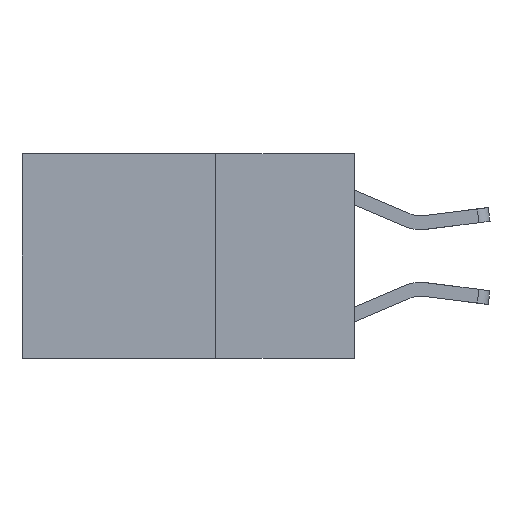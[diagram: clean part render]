
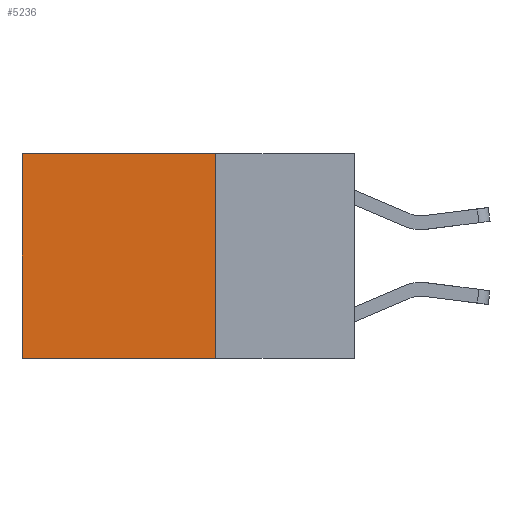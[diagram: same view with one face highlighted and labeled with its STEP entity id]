
A CAD part, left-side view. The second image highlights one B-rep face of the part: STEP entity #5236.
In plain terms, the highlighted planar face has unit normal (-1, 0, 0).
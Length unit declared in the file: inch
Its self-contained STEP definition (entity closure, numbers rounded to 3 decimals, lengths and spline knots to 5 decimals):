
#697 = DIRECTION ( 'NONE',  ( 0., 0., -1. ) ) ;
#700 = CARTESIAN_POINT ( 'NONE',  ( 0.2625, 0.25, 0. ) ) ;
#1028 = CARTESIAN_POINT ( 'NONE',  ( 0.2625, 0.25, 0. ) ) ;
#1201 = ORIENTED_EDGE ( 'NONE', *, *, #4564, .T. ) ;
#1416 = VERTEX_POINT ( 'NONE', #5200 ) ;
#1940 = ORIENTED_EDGE ( 'NONE', *, *, #8384, .F. ) ;
#2010 = VECTOR ( 'NONE', #697, 39.37008 ) ;
#2042 = AXIS2_PLACEMENT_3D ( 'NONE', #700, #9902, #4438 ) ;
#3143 = VECTOR ( 'NONE', #3541, 39.37008 ) ;
#3192 = LINE ( 'NONE', #9416, #2010 ) ;
#3209 = EDGE_CURVE ( 'NONE', #5776, #1416, #3192, .T. ) ;
#3302 = EDGE_CURVE ( 'NONE', #5776, #8707, #9714, .T. ) ;
#3541 = DIRECTION ( 'NONE',  ( 0., 0., -1. ) ) ;
#4438 = DIRECTION ( 'NONE',  ( 0., 0., -1. ) ) ;
#4451 = CARTESIAN_POINT ( 'NONE',  ( 0.2625, 0.6, 0. ) ) ;
#4564 = EDGE_CURVE ( 'NONE', #8707, #8783, #5069, .T. ) ;
#5069 = LINE ( 'NONE', #4451, #3143 ) ;
#5200 = CARTESIAN_POINT ( 'NONE',  ( 0.2625, 0.25, -0.37 ) ) ;
#5236 = ADVANCED_FACE ( 'NONE', ( #7650 ), #10007, .F. ) ;
#5656 = CARTESIAN_POINT ( 'NONE',  ( 0.2625, 0.25, -0.37 ) ) ;
#5776 = VERTEX_POINT ( 'NONE', #1028 ) ;
#5894 = CARTESIAN_POINT ( 'NONE',  ( 0.2625, 0.25, 0. ) ) ;
#6573 = DIRECTION ( 'NONE',  ( 0., 1., 0. ) ) ;
#6886 = DIRECTION ( 'NONE',  ( 0., 1., 0. ) ) ;
#7650 = FACE_OUTER_BOUND ( 'NONE', #8470, .T. ) ;
#7672 = VECTOR ( 'NONE', #6886, 39.37008 ) ;
#7957 = ORIENTED_EDGE ( 'NONE', *, *, #3302, .T. ) ;
#8384 = EDGE_CURVE ( 'NONE', #1416, #8783, #9650, .T. ) ;
#8470 = EDGE_LOOP ( 'NONE', ( #1201, #1940, #8890, #7957 ) ) ;
#8653 = VECTOR ( 'NONE', #6573, 39.37008 ) ;
#8707 = VERTEX_POINT ( 'NONE', #9380 ) ;
#8783 = VERTEX_POINT ( 'NONE', #9536 ) ;
#8890 = ORIENTED_EDGE ( 'NONE', *, *, #3209, .F. ) ;
#9380 = CARTESIAN_POINT ( 'NONE',  ( 0.2625, 0.6, 0. ) ) ;
#9416 = CARTESIAN_POINT ( 'NONE',  ( 0.2625, 0.25, 0. ) ) ;
#9536 = CARTESIAN_POINT ( 'NONE',  ( 0.2625, 0.6, -0.37 ) ) ;
#9650 = LINE ( 'NONE', #5656, #8653 ) ;
#9714 = LINE ( 'NONE', #5894, #7672 ) ;
#9902 = DIRECTION ( 'NONE',  ( 1., 0., 0. ) ) ;
#10007 = PLANE ( 'NONE',  #2042 ) ;
